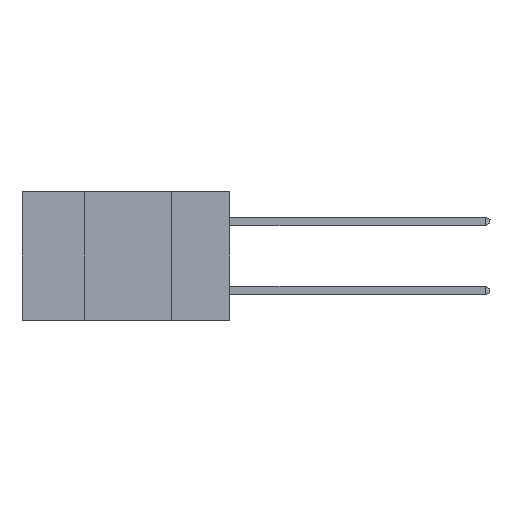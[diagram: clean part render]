
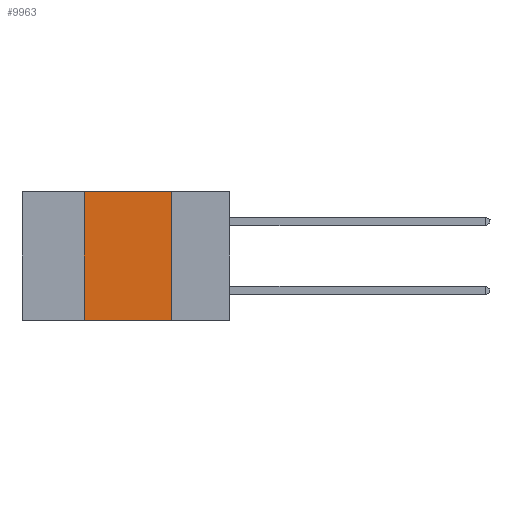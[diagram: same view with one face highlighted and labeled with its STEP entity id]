
A CAD part, left-side view. The second image highlights one B-rep face of the part: STEP entity #9963.
In plain terms, the highlighted planar face has unit normal (-1, 0, 0).
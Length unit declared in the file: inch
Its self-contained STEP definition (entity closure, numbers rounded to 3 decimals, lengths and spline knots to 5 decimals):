
#443 = DIRECTION ( 'NONE',  ( 0., -1., 0. ) ) ;
#491 = CARTESIAN_POINT ( 'NONE',  ( 0., 0.42, -0.37 ) ) ;
#851 = EDGE_CURVE ( 'NONE', #8183, #1519, #10734, .T. ) ;
#1519 = VERTEX_POINT ( 'NONE', #6970 ) ;
#2691 = VECTOR ( 'NONE', #9706, 39.37008 ) ;
#3052 = EDGE_LOOP ( 'NONE', ( #5859, #8090, #5130, #5489 ) ) ;
#3451 = VECTOR ( 'NONE', #443, 39.37008 ) ;
#3998 = VERTEX_POINT ( 'NONE', #491 ) ;
#4740 = CARTESIAN_POINT ( 'NONE',  ( 0., 0.42, 0. ) ) ;
#5130 = ORIENTED_EDGE ( 'NONE', *, *, #7480, .F. ) ;
#5477 = CARTESIAN_POINT ( 'NONE',  ( 0., 0.6, 0. ) ) ;
#5489 = ORIENTED_EDGE ( 'NONE', *, *, #5963, .T. ) ;
#5852 = DIRECTION ( 'NONE',  ( 0., 0., -1. ) ) ;
#5859 = ORIENTED_EDGE ( 'NONE', *, *, #6113, .F. ) ;
#5963 = EDGE_CURVE ( 'NONE', #3998, #7104, #8696, .T. ) ;
#6113 = EDGE_CURVE ( 'NONE', #1519, #7104, #9040, .T. ) ;
#6970 = CARTESIAN_POINT ( 'NONE',  ( 0., 0.17, 0. ) ) ;
#7104 = VERTEX_POINT ( 'NONE', #12206 ) ;
#7450 = AXIS2_PLACEMENT_3D ( 'NONE', #12362, #13579, #12427 ) ;
#7480 = EDGE_CURVE ( 'NONE', #3998, #8183, #12377, .T. ) ;
#7993 = DIRECTION ( 'NONE',  ( 0., 0., 1. ) ) ;
#8090 = ORIENTED_EDGE ( 'NONE', *, *, #851, .F. ) ;
#8112 = FACE_OUTER_BOUND ( 'NONE', #3052, .T. ) ;
#8183 = VERTEX_POINT ( 'NONE', #4740 ) ;
#8696 = LINE ( 'NONE', #8894, #3451 ) ;
#8894 = CARTESIAN_POINT ( 'NONE',  ( 0., 0.6, -0.37 ) ) ;
#9040 = LINE ( 'NONE', #11403, #12945 ) ;
#9706 = DIRECTION ( 'NONE',  ( 0., -1., 0. ) ) ;
#9963 = ADVANCED_FACE ( 'NONE', ( #8112 ), #10275, .F. ) ;
#10275 = PLANE ( 'NONE',  #7450 ) ;
#10293 = CARTESIAN_POINT ( 'NONE',  ( 0., 0.42, -0.37 ) ) ;
#10734 = LINE ( 'NONE', #5477, #2691 ) ;
#11403 = CARTESIAN_POINT ( 'NONE',  ( 0., 0.17, -0.37 ) ) ;
#12206 = CARTESIAN_POINT ( 'NONE',  ( 0., 0.17, -0.37 ) ) ;
#12362 = CARTESIAN_POINT ( 'NONE',  ( 0., 0.6, 0. ) ) ;
#12377 = LINE ( 'NONE', #10293, #12978 ) ;
#12427 = DIRECTION ( 'NONE',  ( 0., 0., -1. ) ) ;
#12945 = VECTOR ( 'NONE', #5852, 39.37008 ) ;
#12978 = VECTOR ( 'NONE', #7993, 39.37008 ) ;
#13579 = DIRECTION ( 'NONE',  ( 1., 0., 0. ) ) ;
